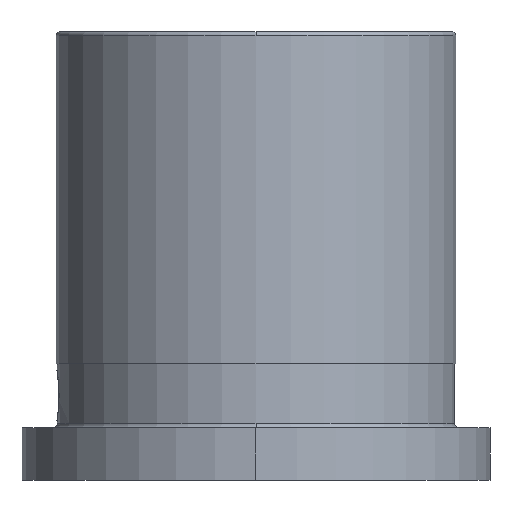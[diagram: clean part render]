
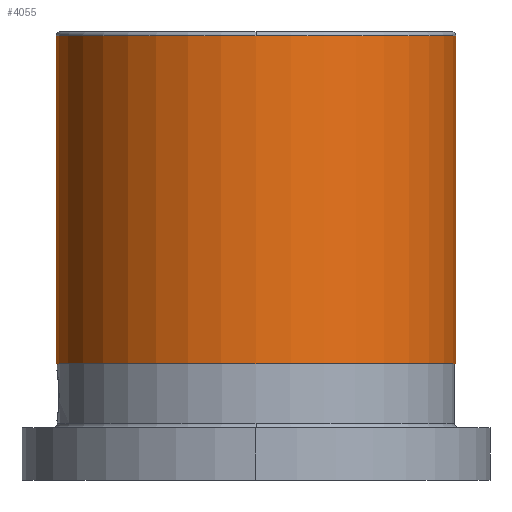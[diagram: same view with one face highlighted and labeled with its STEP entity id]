
A CAD part, left-side view. The second image highlights one B-rep face of the part: STEP entity #4055.
In plain terms, the highlighted cylindrical face has radius 12.684 mm (diameter 25.367 mm), a partial arc.
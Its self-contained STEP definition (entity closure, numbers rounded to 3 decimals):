
#211 = ORIENTED_EDGE ( 'NONE', *, *, #2487, .F. ) ;
#361 = CIRCLE ( 'NONE', #1878, 12.683 ) ;
#390 = LINE ( 'NONE', #3591, #5728 ) ;
#424 = EDGE_CURVE ( 'NONE', #4165, #4747, #390, .T. ) ;
#615 = CARTESIAN_POINT ( 'NONE',  ( 0., 0., 28.219 ) ) ;
#647 = DIRECTION ( 'NONE',  ( 0., 0., 1. ) ) ;
#661 = CARTESIAN_POINT ( 'NONE',  ( -12.683, 0., 28.219 ) ) ;
#730 = ORIENTED_EDGE ( 'NONE', *, *, #2313, .F. ) ;
#849 = CIRCLE ( 'NONE', #2068, 12.683 ) ;
#950 = CARTESIAN_POINT ( 'NONE',  ( 0., 0., 28.219 ) ) ;
#1202 = EDGE_LOOP ( 'NONE', ( #1529, #730, #4423, #211, #1917 ) ) ;
#1252 = DIRECTION ( 'NONE',  ( 0., -1., 0. ) ) ;
#1265 = VERTEX_POINT ( 'NONE', #5488 ) ;
#1529 = ORIENTED_EDGE ( 'NONE', *, *, #2059, .F. ) ;
#1630 = DIRECTION ( 'NONE',  ( 0., 0., 1. ) ) ;
#1799 = DIRECTION ( 'NONE',  ( 0., -1., 0. ) ) ;
#1878 = AXIS2_PLACEMENT_3D ( 'NONE', #615, #4567, #3629 ) ;
#1917 = ORIENTED_EDGE ( 'NONE', *, *, #3167, .F. ) ;
#2059 = EDGE_CURVE ( 'NONE', #1265, #4484, #2407, .T. ) ;
#2068 = AXIS2_PLACEMENT_3D ( 'NONE', #950, #2230, #1799 ) ;
#2078 = FACE_OUTER_BOUND ( 'NONE', #1202, .T. ) ;
#2144 = CIRCLE ( 'NONE', #2901, 12.683 ) ;
#2230 = DIRECTION ( 'NONE',  ( 0., 0., 1. ) ) ;
#2313 = EDGE_CURVE ( 'NONE', #4165, #1265, #2144, .T. ) ;
#2384 = CARTESIAN_POINT ( 'NONE',  ( 0., -12.683, 28.219 ) ) ;
#2407 = LINE ( 'NONE', #4658, #4294 ) ;
#2487 = EDGE_CURVE ( 'NONE', #2881, #4747, #361, .T. ) ;
#2881 = VERTEX_POINT ( 'NONE', #661 ) ;
#2901 = AXIS2_PLACEMENT_3D ( 'NONE', #5800, #4919, #1252 ) ;
#2926 = CARTESIAN_POINT ( 'NONE',  ( 0., -12.683, 7.391 ) ) ;
#3167 = EDGE_CURVE ( 'NONE', #4484, #2881, #849, .T. ) ;
#3464 = AXIS2_PLACEMENT_3D ( 'NONE', #5656, #1630, #5211 ) ;
#3591 = CARTESIAN_POINT ( 'NONE',  ( 0., -12.683, 7.391 ) ) ;
#3629 = DIRECTION ( 'NONE',  ( 0., -1., 0. ) ) ;
#3859 = CYLINDRICAL_SURFACE ( 'NONE', #3464, 12.683 ) ;
#4026 = DIRECTION ( 'NONE',  ( 0., 0., 1. ) ) ;
#4055 = ADVANCED_FACE ( 'NONE', ( #2078 ), #3859, .T. ) ;
#4165 = VERTEX_POINT ( 'NONE', #2926 ) ;
#4294 = VECTOR ( 'NONE', #647, 1000. ) ;
#4401 = CARTESIAN_POINT ( 'NONE',  ( 0., 12.683, 28.219 ) ) ;
#4423 = ORIENTED_EDGE ( 'NONE', *, *, #424, .T. ) ;
#4484 = VERTEX_POINT ( 'NONE', #4401 ) ;
#4567 = DIRECTION ( 'NONE',  ( 0., 0., 1. ) ) ;
#4658 = CARTESIAN_POINT ( 'NONE',  ( 0., 12.683, 7.391 ) ) ;
#4747 = VERTEX_POINT ( 'NONE', #2384 ) ;
#4919 = DIRECTION ( 'NONE',  ( 0., 0., -1. ) ) ;
#5211 = DIRECTION ( 'NONE',  ( 0., -1., 0. ) ) ;
#5488 = CARTESIAN_POINT ( 'NONE',  ( 0., 12.683, 7.391 ) ) ;
#5656 = CARTESIAN_POINT ( 'NONE',  ( 0., 0., 7.391 ) ) ;
#5728 = VECTOR ( 'NONE', #4026, 1000. ) ;
#5800 = CARTESIAN_POINT ( 'NONE',  ( 0., 0., 7.391 ) ) ;
